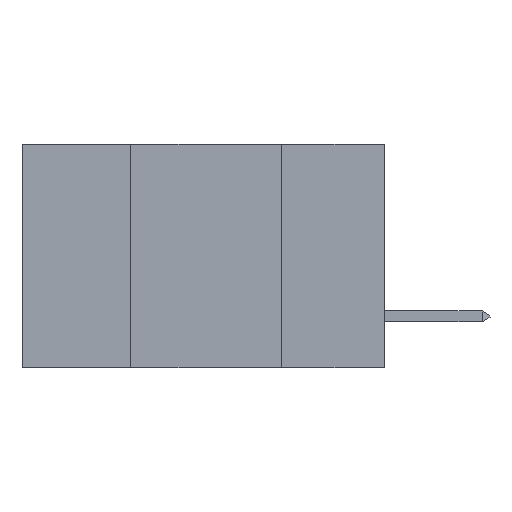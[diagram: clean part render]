
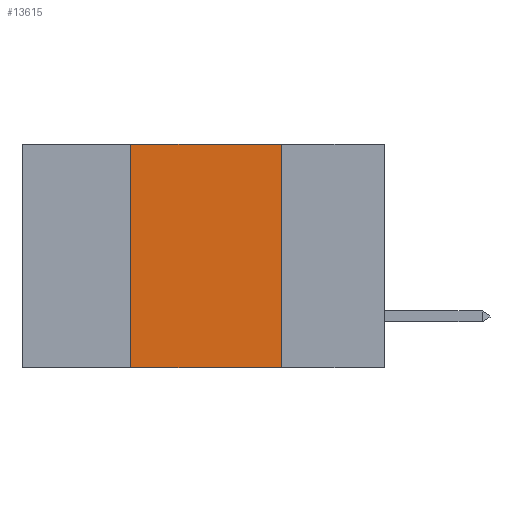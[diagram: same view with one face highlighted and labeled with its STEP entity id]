
A CAD part, left-side view. The second image highlights one B-rep face of the part: STEP entity #13615.
In plain terms, the highlighted planar face has unit normal (-1, 0, 0).
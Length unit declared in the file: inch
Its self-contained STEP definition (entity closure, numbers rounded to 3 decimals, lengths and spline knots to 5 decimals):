
#1330 = VECTOR ( 'NONE', #14223, 39.37008 ) ;
#1566 = DIRECTION ( 'NONE',  ( 0., 0., 1. ) ) ;
#4128 = CARTESIAN_POINT ( 'NONE',  ( 0., 0.42, -0.37 ) ) ;
#5815 = VECTOR ( 'NONE', #1566, 39.37008 ) ;
#6099 = CARTESIAN_POINT ( 'NONE',  ( 0., 0.6, -0.37 ) ) ;
#6326 = CARTESIAN_POINT ( 'NONE',  ( 0., 0.6, 0. ) ) ;
#7242 = ORIENTED_EDGE ( 'NONE', *, *, #13448, .F. ) ;
#7266 = ORIENTED_EDGE ( 'NONE', *, *, #16327, .F. ) ;
#7457 = ORIENTED_EDGE ( 'NONE', *, *, #16241, .T. ) ;
#7685 = CARTESIAN_POINT ( 'NONE',  ( 0., 0.42, 0. ) ) ;
#7883 = VERTEX_POINT ( 'NONE', #4128 ) ;
#8261 = EDGE_CURVE ( 'NONE', #7883, #8472, #18666, .T. ) ;
#8472 = VERTEX_POINT ( 'NONE', #7685 ) ;
#8973 = DIRECTION ( 'NONE',  ( 0., 0., -1. ) ) ;
#9520 = AXIS2_PLACEMENT_3D ( 'NONE', #15321, #18490, #8973 ) ;
#9539 = VECTOR ( 'NONE', #14925, 39.37008 ) ;
#10049 = LINE ( 'NONE', #18022, #9539 ) ;
#10163 = CARTESIAN_POINT ( 'NONE',  ( 0., 0.42, 0. ) ) ;
#10283 = FACE_OUTER_BOUND ( 'NONE', #14142, .T. ) ;
#10813 = CARTESIAN_POINT ( 'NONE',  ( 0., 0.17, 0. ) ) ;
#10981 = CARTESIAN_POINT ( 'NONE',  ( 0., 0.17, -0.37 ) ) ;
#13125 = VERTEX_POINT ( 'NONE', #10981 ) ;
#13448 = EDGE_CURVE ( 'NONE', #13703, #13125, #10049, .T. ) ;
#13615 = ADVANCED_FACE ( 'NONE', ( #10283 ), #13755, .F. ) ;
#13703 = VERTEX_POINT ( 'NONE', #10813 ) ;
#13755 = PLANE ( 'NONE',  #9520 ) ;
#14142 = EDGE_LOOP ( 'NONE', ( #7242, #7266, #21278, #7457 ) ) ;
#14223 = DIRECTION ( 'NONE',  ( 0., -1., 0. ) ) ;
#14925 = DIRECTION ( 'NONE',  ( 0., 0., -1. ) ) ;
#15120 = LINE ( 'NONE', #6099, #1330 ) ;
#15321 = CARTESIAN_POINT ( 'NONE',  ( 0., 0.6, 0. ) ) ;
#16074 = DIRECTION ( 'NONE',  ( 0., -1., 0. ) ) ;
#16241 = EDGE_CURVE ( 'NONE', #7883, #13125, #15120, .T. ) ;
#16327 = EDGE_CURVE ( 'NONE', #8472, #13703, #16829, .T. ) ;
#16829 = LINE ( 'NONE', #6326, #21077 ) ;
#18022 = CARTESIAN_POINT ( 'NONE',  ( 0., 0.17, 0. ) ) ;
#18490 = DIRECTION ( 'NONE',  ( 1., 0., 0. ) ) ;
#18666 = LINE ( 'NONE', #10163, #5815 ) ;
#21077 = VECTOR ( 'NONE', #16074, 39.37008 ) ;
#21278 = ORIENTED_EDGE ( 'NONE', *, *, #8261, .F. ) ;
